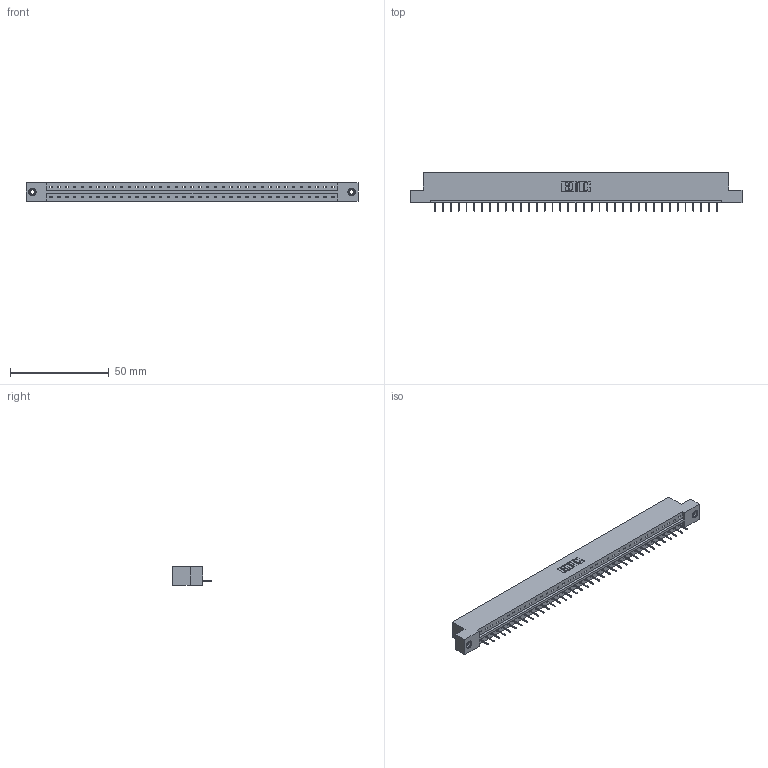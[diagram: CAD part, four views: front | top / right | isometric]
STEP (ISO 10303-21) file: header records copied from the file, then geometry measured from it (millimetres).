
FILE_DESCRIPTION (( 'STEP AP203' ), '1' );
FILE_NAME ('833-037-524-108.STEP', '2020-06-03T05:05:51', ( '' ), ( '' ), 'SwSTEP 2.0', 'SolidWorks 2020', '' );
FILE_SCHEMA (( 'CONFIG_CONTROL_DESIGN' ));
Length unit declared in the file: inch
Products named in the file (4): 345-292-001_345-293-124; 833 Part_Flush - .156 Dia - TI; 833-037-524-108; 345-250-001_345-250-003-102
Assembly tree (40 placements, depth 2):
  833-037-524-108
    833 Part_Flush - .156 Dia - TI
    345-292-001_345-293-124  x37
    345-250-001_345-250-003-102  x2
Bounding box: 168.15 x 19.69 x 9.4 mm (x, y, z)
Volume: 16724.8 mm3; surface area: 17586.7 mm2
Topology: 40 solids, 40 shells, 2468 faces, 7107 edges, 4582 vertices
Faces by surface type: plane 1878, cylinder 574, cone 12, torus 4
Entity records: 24526 total; most frequent: CARTESIAN_POINT 4212, ORIENTED_EDGE 4178, DIRECTION 3597, EDGE_CURVE 2089, LINE 1945, VECTOR 1945, VERTEX_POINT 1384, AXIS2_PLACEMENT_3D 826
